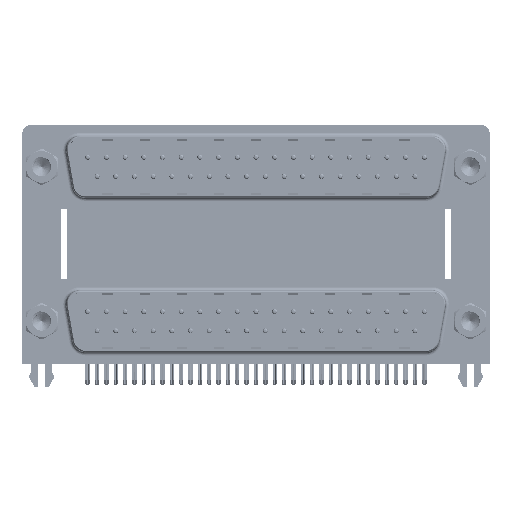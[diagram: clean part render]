
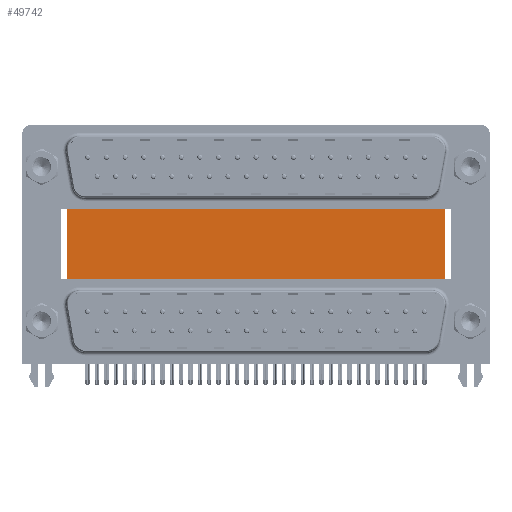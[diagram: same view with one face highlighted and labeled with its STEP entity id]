
A CAD part, top view. The second image highlights one B-rep face of the part: STEP entity #49742.
In plain terms, the highlighted planar face has unit normal (0, 0, 1).
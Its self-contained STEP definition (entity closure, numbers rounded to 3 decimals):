
#1249 = VECTOR ( 'NONE', #32374, 1000. ) ;
#2777 = DIRECTION ( 'NONE',  ( -1., 0., 0. ) ) ;
#3210 = CARTESIAN_POINT ( 'NONE',  ( 3.79, 16.585, -12. ) ) ;
#3489 = LINE ( 'NONE', #21261, #8042 ) ;
#6235 = CARTESIAN_POINT ( 'NONE',  ( 3.79, 16.585, -12. ) ) ;
#6576 = VERTEX_POINT ( 'NONE', #54957 ) ;
#7634 = ORIENTED_EDGE ( 'NONE', *, *, #52902, .T. ) ;
#8042 = VECTOR ( 'NONE', #16899, 1000. ) ;
#8683 = CARTESIAN_POINT ( 'NONE',  ( 59.71, 16.585, -12. ) ) ;
#9638 = EDGE_CURVE ( 'NONE', #21374, #32263, #3489, .T. ) ;
#10951 = DIRECTION ( 'NONE',  ( 0., 0., -1. ) ) ;
#12570 = EDGE_CURVE ( 'NONE', #6576, #32263, #22369, .T. ) ;
#15866 = AXIS2_PLACEMENT_3D ( 'NONE', #19701, #10951, #2777 ) ;
#16531 = ORIENTED_EDGE ( 'NONE', *, *, #48818, .F. ) ;
#16899 = DIRECTION ( 'NONE',  ( 1., 0., 0. ) ) ;
#19701 = CARTESIAN_POINT ( 'NONE',  ( 3.79, 16.585, -12. ) ) ;
#20076 = ORIENTED_EDGE ( 'NONE', *, *, #9638, .T. ) ;
#21261 = CARTESIAN_POINT ( 'NONE',  ( 3.79, -3.735, -12. ) ) ;
#21374 = VERTEX_POINT ( 'NONE', #52469 ) ;
#22369 = LINE ( 'NONE', #8683, #22767 ) ;
#22767 = VECTOR ( 'NONE', #44787, 1000. ) ;
#28134 = VERTEX_POINT ( 'NONE', #6235 ) ;
#29003 = FACE_OUTER_BOUND ( 'NONE', #41826, .T. ) ;
#32263 = VERTEX_POINT ( 'NONE', #49951 ) ;
#32374 = DIRECTION ( 'NONE',  ( 0., -1., 0. ) ) ;
#32435 = ORIENTED_EDGE ( 'NONE', *, *, #12570, .F. ) ;
#32512 = VECTOR ( 'NONE', #56191, 1000. ) ;
#41826 = EDGE_LOOP ( 'NONE', ( #20076, #32435, #16531, #7634 ) ) ;
#42203 = CARTESIAN_POINT ( 'NONE',  ( 3.79, 16.585, -12. ) ) ;
#44787 = DIRECTION ( 'NONE',  ( 0., -1., 0. ) ) ;
#46564 = LINE ( 'NONE', #42203, #1249 ) ;
#48818 = EDGE_CURVE ( 'NONE', #28134, #6576, #55901, .T. ) ;
#49742 = ADVANCED_FACE ( 'NONE', ( #29003 ), #51130, .F. ) ;
#49951 = CARTESIAN_POINT ( 'NONE',  ( 59.71, -3.735, -12. ) ) ;
#51130 = PLANE ( 'NONE',  #15866 ) ;
#52469 = CARTESIAN_POINT ( 'NONE',  ( 3.79, -3.735, -12. ) ) ;
#52902 = EDGE_CURVE ( 'NONE', #28134, #21374, #46564, .T. ) ;
#54957 = CARTESIAN_POINT ( 'NONE',  ( 59.71, 16.585, -12. ) ) ;
#55901 = LINE ( 'NONE', #3210, #32512 ) ;
#56191 = DIRECTION ( 'NONE',  ( 1., 0., 0. ) ) ;
